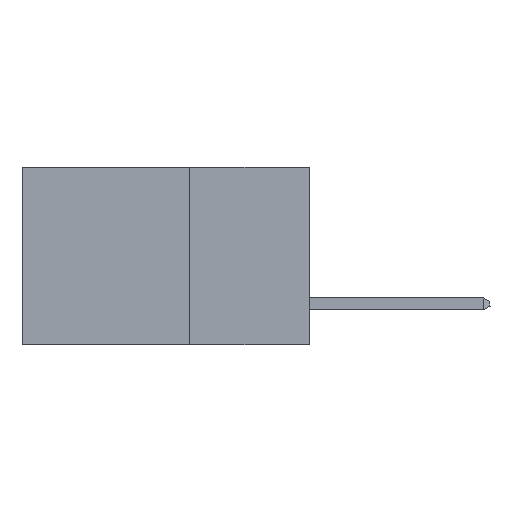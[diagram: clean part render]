
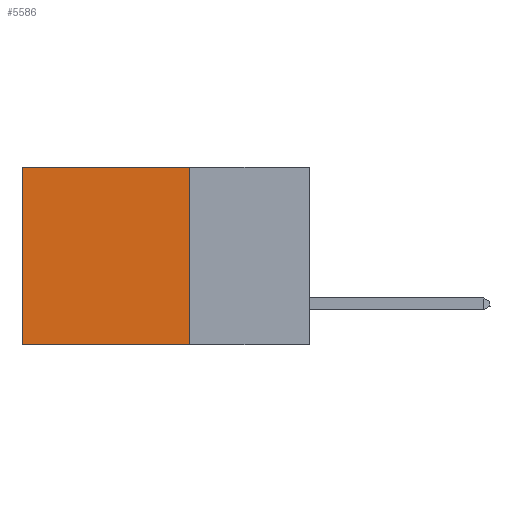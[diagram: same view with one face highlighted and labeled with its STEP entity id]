
A CAD part, left-side view. The second image highlights one B-rep face of the part: STEP entity #5586.
In plain terms, the highlighted planar face has unit normal (-1, 0, 0).
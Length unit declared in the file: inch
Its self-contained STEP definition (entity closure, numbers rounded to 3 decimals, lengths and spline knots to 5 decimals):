
#26 = CARTESIAN_POINT ( 'NONE',  ( 0.2875, 0.6, 0. ) ) ;
#174 = CARTESIAN_POINT ( 'NONE',  ( 0.2875, 0.25, 0. ) ) ;
#945 = ORIENTED_EDGE ( 'NONE', *, *, #9777, .T. ) ;
#1076 = DIRECTION ( 'NONE',  ( 0., 1., 0. ) ) ;
#1111 = EDGE_LOOP ( 'NONE', ( #945, #9763, #4005, #4898 ) ) ;
#1255 = CARTESIAN_POINT ( 'NONE',  ( 0.2875, 0.6, 0. ) ) ;
#1574 = CARTESIAN_POINT ( 'NONE',  ( 0.2875, 0.25, -0.37 ) ) ;
#2092 = DIRECTION ( 'NONE',  ( 1., 0., 0. ) ) ;
#2550 = DIRECTION ( 'NONE',  ( 0., 0., -1. ) ) ;
#2562 = VECTOR ( 'NONE', #7492, 39.37008 ) ;
#3010 = DIRECTION ( 'NONE',  ( 0., 0., -1. ) ) ;
#3157 = LINE ( 'NONE', #174, #2562 ) ;
#3446 = EDGE_CURVE ( 'NONE', #7008, #7814, #7798, .T. ) ;
#3473 = AXIS2_PLACEMENT_3D ( 'NONE', #9378, #2092, #3010 ) ;
#3821 = VECTOR ( 'NONE', #1076, 39.37008 ) ;
#3945 = VERTEX_POINT ( 'NONE', #26 ) ;
#4005 = ORIENTED_EDGE ( 'NONE', *, *, #3446, .F. ) ;
#4898 = ORIENTED_EDGE ( 'NONE', *, *, #7805, .T. ) ;
#5267 = LINE ( 'NONE', #1255, #10395 ) ;
#5586 = ADVANCED_FACE ( 'NONE', ( #6794 ), #11178, .F. ) ;
#6133 = LINE ( 'NONE', #1574, #3821 ) ;
#6794 = FACE_OUTER_BOUND ( 'NONE', #1111, .T. ) ;
#6826 = CARTESIAN_POINT ( 'NONE',  ( 0.2875, 0.25, -0.37 ) ) ;
#7008 = VERTEX_POINT ( 'NONE', #7162 ) ;
#7159 = CARTESIAN_POINT ( 'NONE',  ( 0.2875, 0.25, 0. ) ) ;
#7162 = CARTESIAN_POINT ( 'NONE',  ( 0.2875, 0.25, 0. ) ) ;
#7246 = CARTESIAN_POINT ( 'NONE',  ( 0.2875, 0.6, -0.37 ) ) ;
#7492 = DIRECTION ( 'NONE',  ( 0., 1., 0. ) ) ;
#7798 = LINE ( 'NONE', #7159, #9504 ) ;
#7805 = EDGE_CURVE ( 'NONE', #7008, #3945, #3157, .T. ) ;
#7814 = VERTEX_POINT ( 'NONE', #6826 ) ;
#8450 = VERTEX_POINT ( 'NONE', #7246 ) ;
#9378 = CARTESIAN_POINT ( 'NONE',  ( 0.2875, 0.25, 0. ) ) ;
#9504 = VECTOR ( 'NONE', #2550, 39.37008 ) ;
#9665 = EDGE_CURVE ( 'NONE', #7814, #8450, #6133, .T. ) ;
#9763 = ORIENTED_EDGE ( 'NONE', *, *, #9665, .F. ) ;
#9777 = EDGE_CURVE ( 'NONE', #3945, #8450, #5267, .T. ) ;
#10395 = VECTOR ( 'NONE', #10467, 39.37008 ) ;
#10467 = DIRECTION ( 'NONE',  ( 0., 0., -1. ) ) ;
#11178 = PLANE ( 'NONE',  #3473 ) ;
